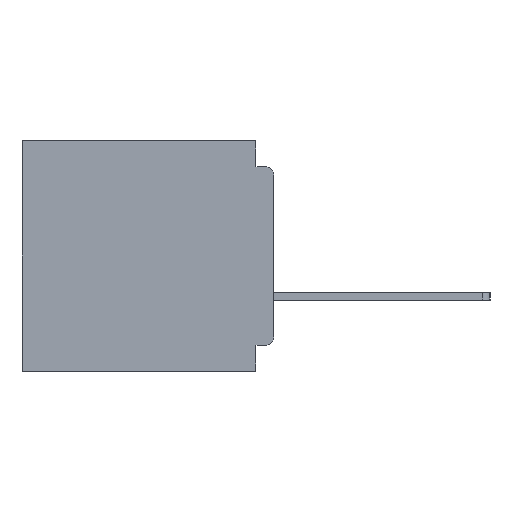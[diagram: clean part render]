
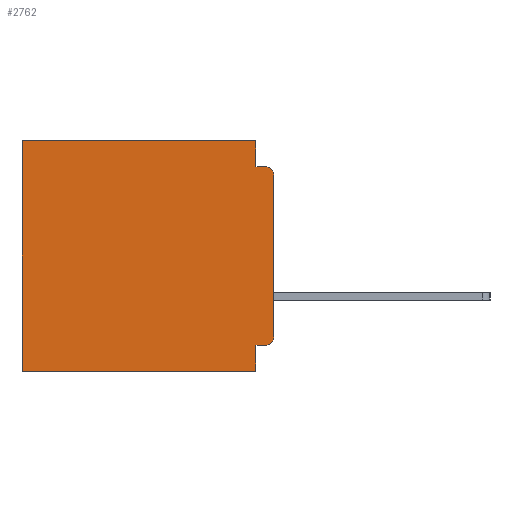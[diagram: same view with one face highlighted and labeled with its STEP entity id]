
A CAD part, left-side view. The second image highlights one B-rep face of the part: STEP entity #2762.
In plain terms, the highlighted planar face has unit normal (-1, 0, 0).
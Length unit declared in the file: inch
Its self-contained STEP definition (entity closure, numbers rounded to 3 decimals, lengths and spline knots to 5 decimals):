
#7 = VERTEX_POINT ( 'NONE', #32804 ) ;
#88 = DIRECTION ( 'NONE',  ( 0., 0., -1. ) ) ;
#648 = CARTESIAN_POINT ( 'NONE',  ( 0.3, 0.031, -0.4 ) ) ;
#721 = ORIENTED_EDGE ( 'NONE', *, *, #14602, .T. ) ;
#1521 = CARTESIAN_POINT ( 'NONE',  ( 0.3, 0.031, 0. ) ) ;
#2352 = DIRECTION ( 'NONE',  ( 0., 0., -1. ) ) ;
#2555 = PLANE ( 'NONE',  #32395 ) ;
#2762 = ADVANCED_FACE ( 'NONE', ( #17481 ), #2555, .F. ) ;
#2918 = CARTESIAN_POINT ( 'NONE',  ( 0.3, 0., 0. ) ) ;
#3727 = DIRECTION ( 'NONE',  ( 1., 0., 0. ) ) ;
#3959 = VERTEX_POINT ( 'NONE', #16250 ) ;
#4377 = DIRECTION ( 'NONE',  ( 0., 0., -1. ) ) ;
#4652 = CARTESIAN_POINT ( 'NONE',  ( 0.3, 0.015, -0.355 ) ) ;
#4749 = CARTESIAN_POINT ( 'NONE',  ( 0.3, 0.015, -0.34 ) ) ;
#6349 = CARTESIAN_POINT ( 'NONE',  ( 0.3, 0.437, 0. ) ) ;
#6939 = VECTOR ( 'NONE', #17793, 39.37008 ) ;
#7338 = ORIENTED_EDGE ( 'NONE', *, *, #18177, .F. ) ;
#7341 = VECTOR ( 'NONE', #4377, 39.37008 ) ;
#7410 = CARTESIAN_POINT ( 'NONE',  ( 0.3, 0.031, 0. ) ) ;
#7522 = DIRECTION ( 'NONE',  ( 0., 0., -1. ) ) ;
#7745 = DIRECTION ( 'NONE',  ( -1., 0., 0. ) ) ;
#7808 = VERTEX_POINT ( 'NONE', #7410 ) ;
#8312 = LINE ( 'NONE', #33055, #14811 ) ;
#8479 = VECTOR ( 'NONE', #20969, 39.37008 ) ;
#10194 = AXIS2_PLACEMENT_3D ( 'NONE', #4749, #24056, #7522 ) ;
#10355 = LINE ( 'NONE', #27510, #15115 ) ;
#10900 = VERTEX_POINT ( 'NONE', #21793 ) ;
#10998 = EDGE_CURVE ( 'NONE', #7808, #34261, #31356, .T. ) ;
#11323 = EDGE_CURVE ( 'NONE', #7808, #15440, #35526, .T. ) ;
#11483 = EDGE_CURVE ( 'NONE', #30021, #18950, #10355, .T. ) ;
#11782 = ORIENTED_EDGE ( 'NONE', *, *, #10998, .T. ) ;
#12430 = VERTEX_POINT ( 'NONE', #4652 ) ;
#12618 = LINE ( 'NONE', #32161, #27187 ) ;
#13104 = ORIENTED_EDGE ( 'NONE', *, *, #24659, .T. ) ;
#13569 = ORIENTED_EDGE ( 'NONE', *, *, #11483, .F. ) ;
#13972 = DIRECTION ( 'NONE',  ( 0., 1., 0. ) ) ;
#14171 = CARTESIAN_POINT ( 'NONE',  ( 0.3, 0.015, -0.045 ) ) ;
#14242 = ORIENTED_EDGE ( 'NONE', *, *, #32917, .F. ) ;
#14602 = EDGE_CURVE ( 'NONE', #3959, #31331, #15892, .T. ) ;
#14811 = VECTOR ( 'NONE', #88, 39.37008 ) ;
#14875 = ORIENTED_EDGE ( 'NONE', *, *, #22453, .F. ) ;
#14988 = CARTESIAN_POINT ( 'NONE',  ( 0.3, 0., -0.045 ) ) ;
#15115 = VECTOR ( 'NONE', #16689, 39.37008 ) ;
#15440 = VERTEX_POINT ( 'NONE', #25627 ) ;
#15869 = DIRECTION ( 'NONE',  ( 0., 1., 0. ) ) ;
#15892 = CIRCLE ( 'NONE', #23142, 0.015 ) ;
#16250 = CARTESIAN_POINT ( 'NONE',  ( 0.3, 0., -0.06 ) ) ;
#16668 = CARTESIAN_POINT ( 'NONE',  ( 0.3, 0.437, -0.4 ) ) ;
#16689 = DIRECTION ( 'NONE',  ( 0., 1., 0. ) ) ;
#17481 = FACE_OUTER_BOUND ( 'NONE', #34061, .T. ) ;
#17793 = DIRECTION ( 'NONE',  ( 0., -1., 0. ) ) ;
#18177 = EDGE_CURVE ( 'NONE', #12430, #7, #12618, .T. ) ;
#18950 = VERTEX_POINT ( 'NONE', #16668 ) ;
#20969 = DIRECTION ( 'NONE',  ( 0., 0., -1. ) ) ;
#20979 = LINE ( 'NONE', #24495, #27317 ) ;
#21587 = ORIENTED_EDGE ( 'NONE', *, *, #35425, .F. ) ;
#21629 = LINE ( 'NONE', #14988, #6939 ) ;
#21793 = CARTESIAN_POINT ( 'NONE',  ( 0.3, 0., -0.34 ) ) ;
#22036 = ORIENTED_EDGE ( 'NONE', *, *, #11323, .F. ) ;
#22453 = EDGE_CURVE ( 'NONE', #7, #30021, #30342, .T. ) ;
#22467 = ORIENTED_EDGE ( 'NONE', *, *, #23940, .T. ) ;
#23142 = AXIS2_PLACEMENT_3D ( 'NONE', #24271, #7745, #26959 ) ;
#23342 = VECTOR ( 'NONE', #13972, 39.37008 ) ;
#23940 = EDGE_CURVE ( 'NONE', #12430, #10900, #26858, .T. ) ;
#24056 = DIRECTION ( 'NONE',  ( -1., 0., 0. ) ) ;
#24271 = CARTESIAN_POINT ( 'NONE',  ( 0.3, 0.015, -0.06 ) ) ;
#24380 = DIRECTION ( 'NONE',  ( 0., 0., -1. ) ) ;
#24495 = CARTESIAN_POINT ( 'NONE',  ( 0.3, 0., -0.4 ) ) ;
#24659 = EDGE_CURVE ( 'NONE', #34261, #18950, #8312, .T. ) ;
#25627 = CARTESIAN_POINT ( 'NONE',  ( 0.3, 0.031, -0.045 ) ) ;
#26858 = CIRCLE ( 'NONE', #10194, 0.015 ) ;
#26959 = DIRECTION ( 'NONE',  ( 0., 0., -1. ) ) ;
#27187 = VECTOR ( 'NONE', #15869, 39.37008 ) ;
#27317 = VECTOR ( 'NONE', #24380, 39.37008 ) ;
#27510 = CARTESIAN_POINT ( 'NONE',  ( 0.3, 0., -0.4 ) ) ;
#29138 = CARTESIAN_POINT ( 'NONE',  ( 0.3, 0.031, -0.4 ) ) ;
#30021 = VERTEX_POINT ( 'NONE', #648 ) ;
#30342 = LINE ( 'NONE', #29138, #8479 ) ;
#31331 = VERTEX_POINT ( 'NONE', #14171 ) ;
#31356 = LINE ( 'NONE', #2918, #23342 ) ;
#32161 = CARTESIAN_POINT ( 'NONE',  ( 0.3, 0., -0.355 ) ) ;
#32395 = AXIS2_PLACEMENT_3D ( 'NONE', #32878, #3727, #2352 ) ;
#32804 = CARTESIAN_POINT ( 'NONE',  ( 0.3, 0.031, -0.355 ) ) ;
#32878 = CARTESIAN_POINT ( 'NONE',  ( 0.3, 0., -0.4 ) ) ;
#32917 = EDGE_CURVE ( 'NONE', #3959, #10900, #20979, .T. ) ;
#33055 = CARTESIAN_POINT ( 'NONE',  ( 0.3, 0.437, -0.4 ) ) ;
#34061 = EDGE_LOOP ( 'NONE', ( #14242, #721, #21587, #22036, #11782, #13104, #13569, #14875, #7338, #22467 ) ) ;
#34261 = VERTEX_POINT ( 'NONE', #6349 ) ;
#35425 = EDGE_CURVE ( 'NONE', #15440, #31331, #21629, .T. ) ;
#35526 = LINE ( 'NONE', #1521, #7341 ) ;
